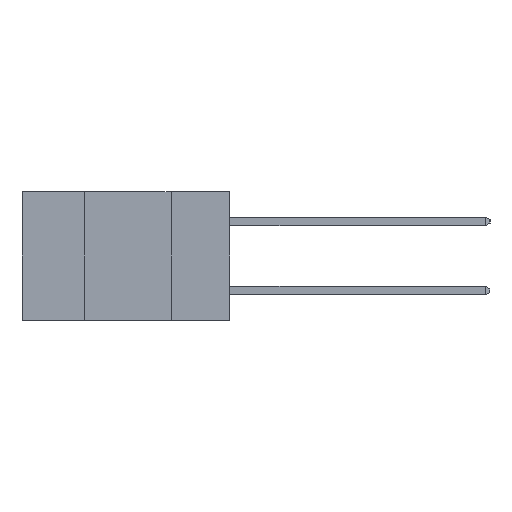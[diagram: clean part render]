
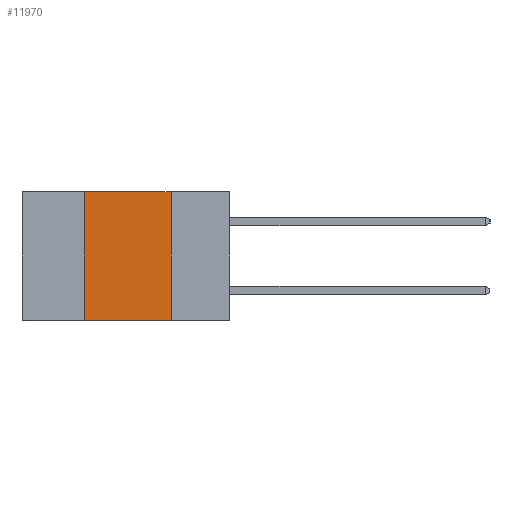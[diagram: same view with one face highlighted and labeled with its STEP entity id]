
A CAD part, left-side view. The second image highlights one B-rep face of the part: STEP entity #11970.
In plain terms, the highlighted planar face has unit normal (-1, 0, 0).
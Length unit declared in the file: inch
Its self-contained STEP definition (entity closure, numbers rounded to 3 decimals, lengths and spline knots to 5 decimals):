
#460 = EDGE_LOOP ( 'NONE', ( #18323, #15397, #11643, #12973 ) ) ;
#1723 = VECTOR ( 'NONE', #27776, 39.37008 ) ;
#2032 = CARTESIAN_POINT ( 'NONE',  ( 0., 0.6, -0.37 ) ) ;
#3173 = VERTEX_POINT ( 'NONE', #27560 ) ;
#3476 = VERTEX_POINT ( 'NONE', #24223 ) ;
#3644 = PLANE ( 'NONE',  #26984 ) ;
#4242 = DIRECTION ( 'NONE',  ( 0., -1., 0. ) ) ;
#4324 = VECTOR ( 'NONE', #4242, 39.37008 ) ;
#6027 = CARTESIAN_POINT ( 'NONE',  ( 0., 0.17, 0. ) ) ;
#6624 = VECTOR ( 'NONE', #27287, 39.37008 ) ;
#6747 = VECTOR ( 'NONE', #25070, 39.37008 ) ;
#10301 = EDGE_CURVE ( 'NONE', #3173, #3476, #18514, .T. ) ;
#10310 = DIRECTION ( 'NONE',  ( 0., 0., -1. ) ) ;
#10335 = CARTESIAN_POINT ( 'NONE',  ( 0., 0.17, -0.37 ) ) ;
#11643 = ORIENTED_EDGE ( 'NONE', *, *, #10301, .F. ) ;
#11970 = ADVANCED_FACE ( 'NONE', ( #16686 ), #3644, .F. ) ;
#12973 = ORIENTED_EDGE ( 'NONE', *, *, #13509, .T. ) ;
#13367 = VERTEX_POINT ( 'NONE', #10335 ) ;
#13463 = LINE ( 'NONE', #16863, #1723 ) ;
#13509 = EDGE_CURVE ( 'NONE', #3173, #13367, #21925, .T. ) ;
#15397 = ORIENTED_EDGE ( 'NONE', *, *, #27728, .F. ) ;
#16686 = FACE_OUTER_BOUND ( 'NONE', #460, .T. ) ;
#16863 = CARTESIAN_POINT ( 'NONE',  ( 0., 0.6, 0. ) ) ;
#18323 = ORIENTED_EDGE ( 'NONE', *, *, #20099, .F. ) ;
#18397 = LINE ( 'NONE', #25117, #6624 ) ;
#18514 = LINE ( 'NONE', #20645, #6747 ) ;
#20099 = EDGE_CURVE ( 'NONE', #20342, #13367, #18397, .T. ) ;
#20342 = VERTEX_POINT ( 'NONE', #6027 ) ;
#20645 = CARTESIAN_POINT ( 'NONE',  ( 0., 0.42, 0. ) ) ;
#21298 = CARTESIAN_POINT ( 'NONE',  ( 0., 0.6, 0. ) ) ;
#21925 = LINE ( 'NONE', #2032, #4324 ) ;
#23525 = DIRECTION ( 'NONE',  ( 1., 0., 0. ) ) ;
#24223 = CARTESIAN_POINT ( 'NONE',  ( 0., 0.42, 0. ) ) ;
#25070 = DIRECTION ( 'NONE',  ( 0., 0., 1. ) ) ;
#25117 = CARTESIAN_POINT ( 'NONE',  ( 0., 0.17, 0. ) ) ;
#26984 = AXIS2_PLACEMENT_3D ( 'NONE', #21298, #23525, #10310 ) ;
#27287 = DIRECTION ( 'NONE',  ( 0., 0., -1. ) ) ;
#27560 = CARTESIAN_POINT ( 'NONE',  ( 0., 0.42, -0.37 ) ) ;
#27728 = EDGE_CURVE ( 'NONE', #3476, #20342, #13463, .T. ) ;
#27776 = DIRECTION ( 'NONE',  ( 0., -1., 0. ) ) ;
